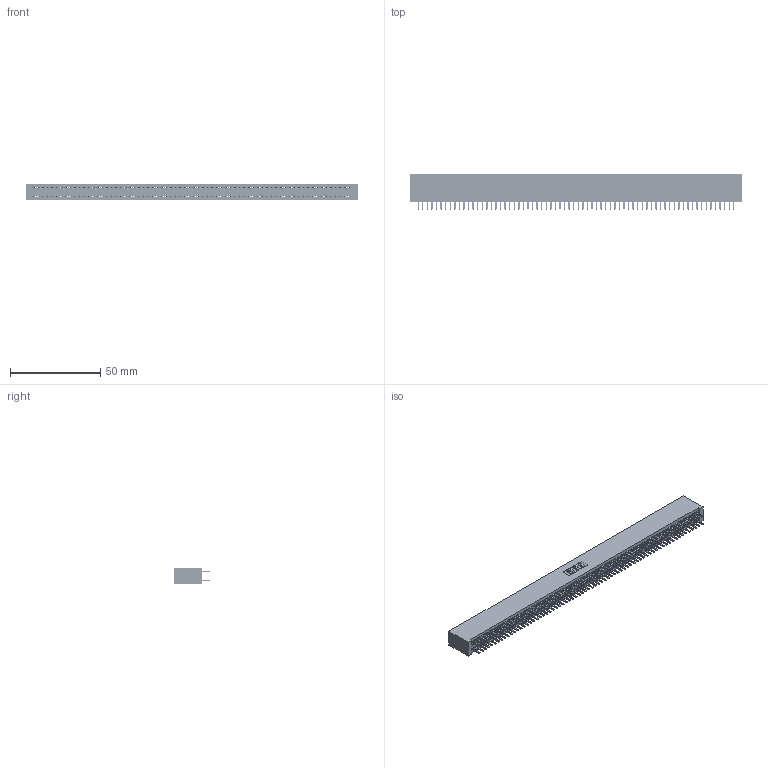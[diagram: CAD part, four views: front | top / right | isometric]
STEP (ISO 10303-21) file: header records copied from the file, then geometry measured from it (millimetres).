
FILE_DESCRIPTION (( 'STEP AP203' ), '1' );
FILE_NAME ('395-140-520-201.STEP', '2018-12-05T19:02:49', ( '' ), ( '' ), 'SwSTEP 2.0', 'SolidWorks 2016', '' );
FILE_SCHEMA (( 'CONFIG_CONTROL_DESIGN' ));
Length unit declared in the file: inch
Products named in the file (3): 395-140-520-201; 345-292-001_345-293-120; 345 Part_No Mounting Lugs
Assembly tree (141 placements, depth 2):
  395-140-520-201
    345 Part_No Mounting Lugs
    345-292-001_345-293-120  x140
Bounding box: 184.4 x 19.68 x 9.4 mm (x, y, z)
Volume: 18727.5 mm3; surface area: 28397 mm2
Topology: 141 solids, 141 shells, 7678 faces, 22297 edges, 14490 vertices
Faces by surface type: plane 4976, cylinder 2702
Entity records: 50991 total; most frequent: CARTESIAN_POINT 8532, ORIENTED_EDGE 8454, DIRECTION 7471, EDGE_CURVE 4227, LINE 3819, VECTOR 3819, VERTEX_POINT 2814, AXIS2_PLACEMENT_3D 1826
